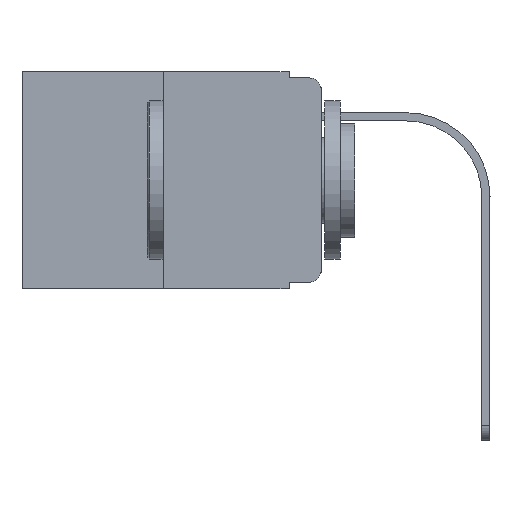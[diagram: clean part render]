
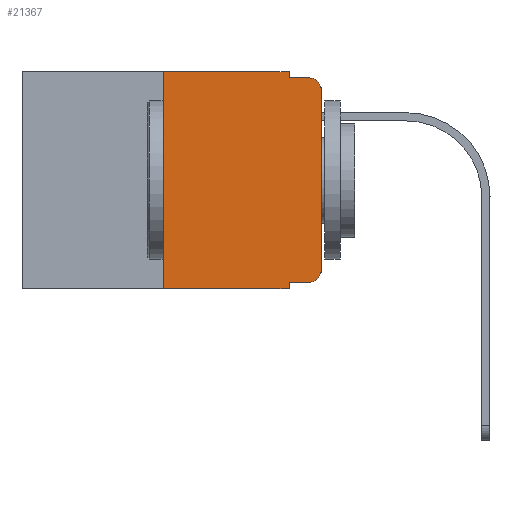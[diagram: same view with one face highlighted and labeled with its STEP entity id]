
A CAD part, left-side view. The second image highlights one B-rep face of the part: STEP entity #21367.
In plain terms, the highlighted planar face has unit normal (-1, 0, 0).
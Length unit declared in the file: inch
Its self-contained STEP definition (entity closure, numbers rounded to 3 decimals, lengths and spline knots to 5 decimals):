
#95 = VERTEX_POINT ( 'NONE', #14791 ) ;
#1197 = LINE ( 'NONE', #21682, #8460 ) ;
#1545 = CIRCLE ( 'NONE', #7717, 0.02 ) ;
#1692 = EDGE_CURVE ( 'NONE', #8986, #7850, #12614, .T. ) ;
#1761 = VERTEX_POINT ( 'NONE', #4744 ) ;
#1779 = CARTESIAN_POINT ( 'NONE',  ( 0., 0.25, -0.343 ) ) ;
#1883 = CARTESIAN_POINT ( 'NONE',  ( 0., 0.051, 0. ) ) ;
#2529 = VECTOR ( 'NONE', #11666, 39.37008 ) ;
#3541 = DIRECTION ( 'NONE',  ( 0., -1., 0. ) ) ;
#4162 = LINE ( 'NONE', #20548, #23706 ) ;
#4280 = CARTESIAN_POINT ( 'NONE',  ( 0., 0.051, -0.333 ) ) ;
#4731 = ORIENTED_EDGE ( 'NONE', *, *, #15417, .F. ) ;
#4744 = CARTESIAN_POINT ( 'NONE',  ( 0., 0.051, -0.01 ) ) ;
#4989 = LINE ( 'NONE', #21845, #7496 ) ;
#5363 = FACE_OUTER_BOUND ( 'NONE', #15828, .T. ) ;
#5570 = CARTESIAN_POINT ( 'NONE',  ( 0., 0.02, -0.03 ) ) ;
#6146 = ORIENTED_EDGE ( 'NONE', *, *, #8792, .F. ) ;
#7288 = LINE ( 'NONE', #1883, #10434 ) ;
#7293 = EDGE_CURVE ( 'NONE', #9763, #20602, #23306, .T. ) ;
#7410 = PLANE ( 'NONE',  #9853 ) ;
#7496 = VECTOR ( 'NONE', #3541, 39.37008 ) ;
#7717 = AXIS2_PLACEMENT_3D ( 'NONE', #22804, #9937, #22916 ) ;
#7850 = VERTEX_POINT ( 'NONE', #21899 ) ;
#8057 = CARTESIAN_POINT ( 'NONE',  ( 0., 0., -0.313 ) ) ;
#8326 = EDGE_CURVE ( 'NONE', #1761, #20688, #4162, .T. ) ;
#8369 = CARTESIAN_POINT ( 'NONE',  ( 0., 0., -0.03 ) ) ;
#8460 = VECTOR ( 'NONE', #23260, 39.37008 ) ;
#8490 = VECTOR ( 'NONE', #22965, 39.37008 ) ;
#8722 = DIRECTION ( 'NONE',  ( 0., -1., 0. ) ) ;
#8792 = EDGE_CURVE ( 'NONE', #19767, #8986, #15380, .T. ) ;
#8986 = VERTEX_POINT ( 'NONE', #16330 ) ;
#9169 = CARTESIAN_POINT ( 'NONE',  ( 0., 0.02, -0.333 ) ) ;
#9763 = VERTEX_POINT ( 'NONE', #23080 ) ;
#9853 = AXIS2_PLACEMENT_3D ( 'NONE', #12642, #13118, #10707 ) ;
#9937 = DIRECTION ( 'NONE',  ( -1., 0., 0. ) ) ;
#10109 = LINE ( 'NONE', #15546, #8490 ) ;
#10434 = VECTOR ( 'NONE', #20294, 39.37008 ) ;
#10707 = DIRECTION ( 'NONE',  ( 0., 0., -1. ) ) ;
#10912 = VERTEX_POINT ( 'NONE', #8057 ) ;
#11226 = ORIENTED_EDGE ( 'NONE', *, *, #8326, .F. ) ;
#11488 = CARTESIAN_POINT ( 'NONE',  ( 0., 0.02, -0.01 ) ) ;
#11666 = DIRECTION ( 'NONE',  ( 0., -1., 0. ) ) ;
#11864 = VECTOR ( 'NONE', #8722, 39.37008 ) ;
#11881 = EDGE_CURVE ( 'NONE', #10912, #19776, #1197, .T. ) ;
#12614 = LINE ( 'NONE', #18069, #11864 ) ;
#12642 = CARTESIAN_POINT ( 'NONE',  ( 0., 0.473, 0. ) ) ;
#12740 = ORIENTED_EDGE ( 'NONE', *, *, #1692, .F. ) ;
#12966 = DIRECTION ( 'NONE',  ( -1., 0., 0. ) ) ;
#13007 = DIRECTION ( 'NONE',  ( 0., -1., 0. ) ) ;
#13118 = DIRECTION ( 'NONE',  ( 1., 0., 0. ) ) ;
#13624 = AXIS2_PLACEMENT_3D ( 'NONE', #5570, #12966, #20750 ) ;
#14436 = ORIENTED_EDGE ( 'NONE', *, *, #14593, .T. ) ;
#14593 = EDGE_CURVE ( 'NONE', #19776, #20688, #21401, .T. ) ;
#14791 = CARTESIAN_POINT ( 'NONE',  ( 0., 0.051, -0.343 ) ) ;
#15159 = EDGE_CURVE ( 'NONE', #7850, #1761, #10109, .T. ) ;
#15380 = LINE ( 'NONE', #22806, #21042 ) ;
#15417 = EDGE_CURVE ( 'NONE', #9763, #95, #7288, .T. ) ;
#15546 = CARTESIAN_POINT ( 'NONE',  ( 0., 0.051, 0. ) ) ;
#15614 = DIRECTION ( 'NONE',  ( 0., 0., 1. ) ) ;
#15828 = EDGE_LOOP ( 'NONE', ( #19818, #14436, #11226, #22639, #12740, #6146, #16647, #4731, #23029, #20617 ) ) ;
#16111 = EDGE_CURVE ( 'NONE', #20602, #10912, #1545, .T. ) ;
#16330 = CARTESIAN_POINT ( 'NONE',  ( 0., 0.25, 0. ) ) ;
#16647 = ORIENTED_EDGE ( 'NONE', *, *, #23015, .T. ) ;
#18069 = CARTESIAN_POINT ( 'NONE',  ( 0., 0.473, 0. ) ) ;
#19767 = VERTEX_POINT ( 'NONE', #1779 ) ;
#19776 = VERTEX_POINT ( 'NONE', #8369 ) ;
#19818 = ORIENTED_EDGE ( 'NONE', *, *, #11881, .T. ) ;
#20294 = DIRECTION ( 'NONE',  ( 0., 0., -1. ) ) ;
#20548 = CARTESIAN_POINT ( 'NONE',  ( 0., 0.051, -0.01 ) ) ;
#20602 = VERTEX_POINT ( 'NONE', #9169 ) ;
#20617 = ORIENTED_EDGE ( 'NONE', *, *, #16111, .T. ) ;
#20688 = VERTEX_POINT ( 'NONE', #11488 ) ;
#20750 = DIRECTION ( 'NONE',  ( 0., 0., -1. ) ) ;
#21042 = VECTOR ( 'NONE', #15614, 39.37008 ) ;
#21367 = ADVANCED_FACE ( 'NONE', ( #5363 ), #7410, .F. ) ;
#21401 = CIRCLE ( 'NONE', #13624, 0.02 ) ;
#21682 = CARTESIAN_POINT ( 'NONE',  ( 0., 0., 0. ) ) ;
#21845 = CARTESIAN_POINT ( 'NONE',  ( 0., 0.473, -0.343 ) ) ;
#21899 = CARTESIAN_POINT ( 'NONE',  ( 0., 0.051, 0. ) ) ;
#22639 = ORIENTED_EDGE ( 'NONE', *, *, #15159, .F. ) ;
#22804 = CARTESIAN_POINT ( 'NONE',  ( 0., 0.02, -0.313 ) ) ;
#22806 = CARTESIAN_POINT ( 'NONE',  ( 0., 0.25, 0. ) ) ;
#22916 = DIRECTION ( 'NONE',  ( 0., 0., -1. ) ) ;
#22965 = DIRECTION ( 'NONE',  ( 0., 0., -1. ) ) ;
#23015 = EDGE_CURVE ( 'NONE', #19767, #95, #4989, .T. ) ;
#23029 = ORIENTED_EDGE ( 'NONE', *, *, #7293, .T. ) ;
#23080 = CARTESIAN_POINT ( 'NONE',  ( 0., 0.051, -0.333 ) ) ;
#23260 = DIRECTION ( 'NONE',  ( 0., 0., 1. ) ) ;
#23306 = LINE ( 'NONE', #4280, #2529 ) ;
#23706 = VECTOR ( 'NONE', #13007, 39.37008 ) ;
